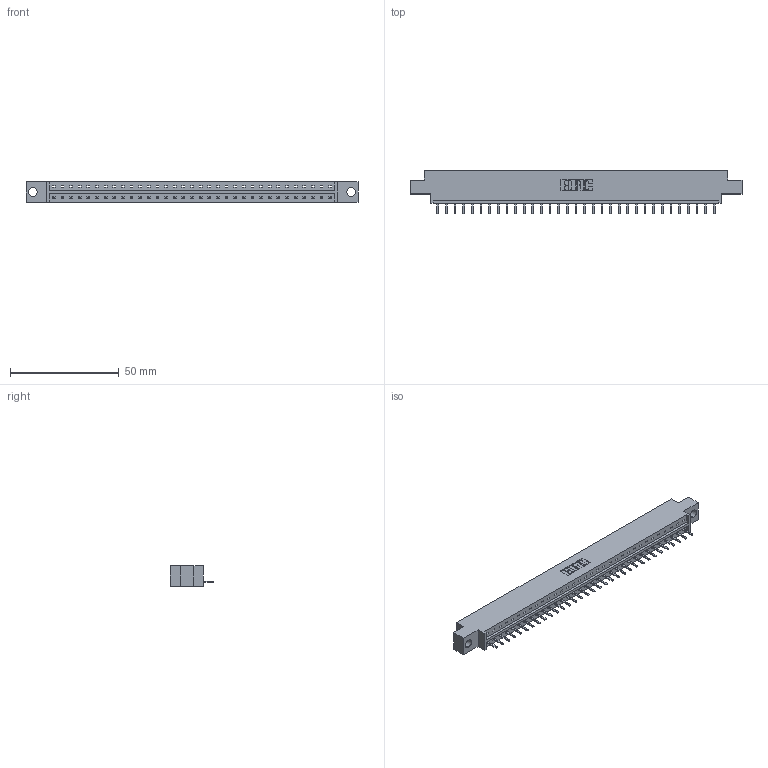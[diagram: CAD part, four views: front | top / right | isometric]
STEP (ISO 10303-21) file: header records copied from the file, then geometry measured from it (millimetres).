
FILE_DESCRIPTION (( 'STEP AP203' ), '1' );
FILE_NAME ('833-033-520-604.STEP', '2020-06-02T19:49:37', ( '' ), ( '' ), 'SwSTEP 2.0', 'SolidWorks 2020', '' );
FILE_SCHEMA (( 'CONFIG_CONTROL_DESIGN' ));
Length unit declared in the file: inch
Products named in the file (3): 345-292-001_345-293-120; 833-033-520-604; 833 Part_Offset - .156 Dia - TH
Assembly tree (34 placements, depth 2):
  833-033-520-604
    833 Part_Offset - .156 Dia - TH
    345-292-001_345-293-120  x33
Bounding box: 152.3 x 20.02 x 9.4 mm (x, y, z)
Volume: 14837.5 mm3; surface area: 15655.4 mm2
Topology: 34 solids, 34 shells, 2164 faces, 6395 edges, 4174 vertices
Faces by surface type: plane 1526, cylinder 638
Entity records: 21587 total; most frequent: CARTESIAN_POINT 3745, ORIENTED_EDGE 3702, DIRECTION 3165, EDGE_CURVE 1851, LINE 1719, VECTOR 1719, VERTEX_POINT 1230, AXIS2_PLACEMENT_3D 723
